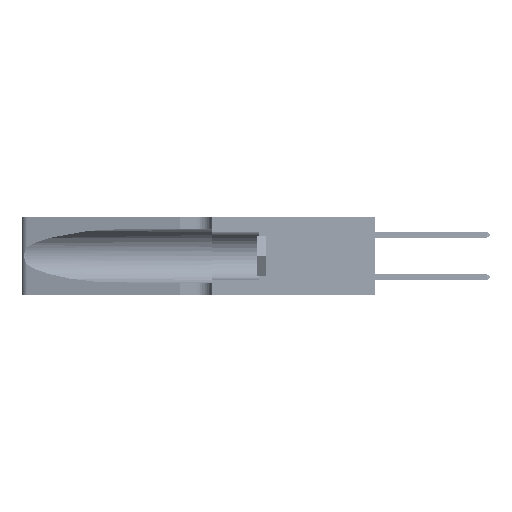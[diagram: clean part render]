
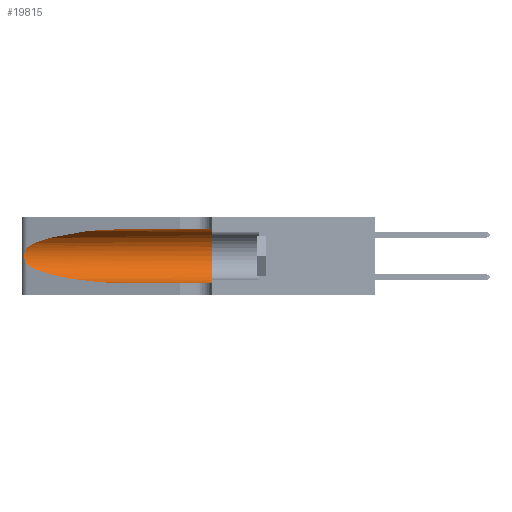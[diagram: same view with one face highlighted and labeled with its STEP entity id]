
A CAD part, left-side view. The second image highlights one B-rep face of the part: STEP entity #19815.
In plain terms, the highlighted cylindrical face has radius 3.308 mm (diameter 6.617 mm), a partial arc.
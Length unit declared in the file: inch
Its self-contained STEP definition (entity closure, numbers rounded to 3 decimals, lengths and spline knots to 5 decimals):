
#216 = DIRECTION ( 'NONE',  ( 0., -1., 0. ) ) ;
#1273 = DIRECTION ( 'NONE',  ( 0., 1., 0. ) ) ;
#1536 = FACE_OUTER_BOUND ( 'NONE', #24089, .T. ) ;
#1923 = VECTOR ( 'NONE', #216, 39.37008 ) ;
#2223 = DIRECTION ( 'NONE',  ( 0., 0., -1. ) ) ;
#2346 = ORIENTED_EDGE ( 'NONE', *, *, #18407, .T. ) ;
#3426 = CARTESIAN_POINT ( 'NONE',  ( 0.25856, 1.23593, 0.16098 ) ) ;
#3861 = CARTESIAN_POINT ( 'NONE',  ( 0.1305, 0.72297, 0.31525 ) ) ;
#4225 = VECTOR ( 'NONE', #5225, 39.37008 ) ;
#5225 = DIRECTION ( 'NONE',  ( 0., -1., 0. ) ) ;
#5783 = LINE ( 'NONE', #40369, #1923 ) ;
#5882 = CARTESIAN_POINT ( 'NONE',  ( 0.1305, 0.72297, 0.05475 ) ) ;
#7433 = VERTEX_POINT ( 'NONE', #36911 ) ;
#7552 = CARTESIAN_POINT ( 'NONE',  ( 0.25639, 1.23186, 0.15144 ) ) ;
#8198 = EDGE_CURVE ( 'NONE', #29718, #7433, #35538, .T. ) ;
#9983 = CARTESIAN_POINT ( 'NONE',  ( 0.25487, 1.22718, 0.22369 ) ) ;
#10720 =( BOUNDED_CURVE ( )  B_SPLINE_CURVE ( 3, ( #15222, #39487, #15399, #43475 ),
 .UNSPECIFIED., .F., .F. ) 
 B_SPLINE_CURVE_WITH_KNOTS ( ( 4, 4 ),
 ( 1.5708, 2.84003 ),
 .UNSPECIFIED. ) 
 CURVE ( )  GEOMETRIC_REPRESENTATION_ITEM ( )  RATIONAL_B_SPLINE_CURVE ( ( 1., 0.87, 0.87, 1. ) ) 
 REPRESENTATION_ITEM ( '' )  );
#11476 = CARTESIAN_POINT ( 'NONE',  ( 0.25487, 1.22718, 0.22369 ) ) ;
#11656 = CARTESIAN_POINT ( 'NONE',  ( 0.25487, 1.22718, 0.14631 ) ) ;
#13279 = AXIS2_PLACEMENT_3D ( 'NONE', #25658, #1273, #29694 ) ;
#13698 = VERTEX_POINT ( 'NONE', #19667 ) ;
#15124 = LINE ( 'NONE', #17372, #4225 ) ;
#15222 = CARTESIAN_POINT ( 'NONE',  ( 0.1305, 0.72297, 0.31525 ) ) ;
#15399 = CARTESIAN_POINT ( 'NONE',  ( 0.2373, 1.15595, 0.28018 ) ) ;
#15605 = CARTESIAN_POINT ( 'NONE',  ( 0.25639, 1.23184, 0.21858 ) ) ;
#15612 = VERTEX_POINT ( 'NONE', #51389 ) ;
#17372 = CARTESIAN_POINT ( 'NONE',  ( 0.1305, 1.61858, 0.05475 ) ) ;
#18407 = EDGE_CURVE ( 'NONE', #13698, #7433, #15124, .T. ) ;
#19667 = CARTESIAN_POINT ( 'NONE',  ( 0.1305, 0.72297, 0.05475 ) ) ;
#19693 = CARTESIAN_POINT ( 'NONE',  ( 0.25854, 1.2359, 0.20912 ) ) ;
#19815 = ADVANCED_FACE ( 'NONE', ( #1536 ), #32636, .F. ) ;
#20430 = ORIENTED_EDGE ( 'NONE', *, *, #29155, .T. ) ;
#21500 = AXIS2_PLACEMENT_3D ( 'NONE', #26624, #22557, #2223 ) ;
#22557 = DIRECTION ( 'NONE',  ( 0., -1., 0. ) ) ;
#23776 = CARTESIAN_POINT ( 'NONE',  ( 0.26075, 1.23896, 0.19203 ) ) ;
#24089 = EDGE_LOOP ( 'NONE', ( #20430, #48212, #42103, #2346, #38307, #40735 ) ) ;
#25658 = CARTESIAN_POINT ( 'NONE',  ( 0.1305, 0.35, 0.185 ) ) ;
#26624 = CARTESIAN_POINT ( 'NONE',  ( 0.1305, 1.61858, 0.185 ) ) ;
#26874 = CARTESIAN_POINT ( 'NONE',  ( 0.1305, 0.35, 0.31525 ) ) ;
#27804 = CARTESIAN_POINT ( 'NONE',  ( 0.26017, 1.23833, 0.17102 ) ) ;
#28047 = VERTEX_POINT ( 'NONE', #3861 ) ;
#29155 = EDGE_CURVE ( 'NONE', #28047, #33355, #10720, .T. ) ;
#29694 = DIRECTION ( 'NONE',  ( 0., 0., 1. ) ) ;
#29718 = VERTEX_POINT ( 'NONE', #26874 ) ;
#30181 = CARTESIAN_POINT ( 'NONE',  ( 0.18966, 0.96281, 0.05475 ) ) ;
#31839 = CARTESIAN_POINT ( 'NONE',  ( 0.25789, 1.23486, 0.15765 ) ) ;
#32636 = CYLINDRICAL_SURFACE ( 'NONE', #21500, 0.13025 ) ;
#33355 = VERTEX_POINT ( 'NONE', #9983 ) ;
#35024 = B_SPLINE_CURVE_WITH_KNOTS ( 'NONE', 3,
 ( #11476, #35686, #15605, #43685, #19693, #47702, #23776, #51707, #27804, #3426, #31839, #7552, #35840, #11656 ),
 .UNSPECIFIED., .F., .F.,
 ( 4, 2, 2, 2, 2, 2, 4 ),
 ( 0., 0.00027, 0.00053, 0.00107, 0.0016, 0.00187, 0.00214 ),
 .UNSPECIFIED. ) ;
#35538 = CIRCLE ( 'NONE', #13279, 0.13025 ) ;
#35686 = CARTESIAN_POINT ( 'NONE',  ( 0.25555, 1.22994, 0.2215 ) ) ;
#35840 = CARTESIAN_POINT ( 'NONE',  ( 0.25555, 1.22993, 0.14849 ) ) ;
#36911 = CARTESIAN_POINT ( 'NONE',  ( 0.1305, 0.35, 0.05475 ) ) ;
#37035 = EDGE_CURVE ( 'NONE', #28047, #29718, #5783, .T. ) ;
#38307 = ORIENTED_EDGE ( 'NONE', *, *, #8198, .F. ) ;
#39487 = CARTESIAN_POINT ( 'NONE',  ( 0.18966, 0.96281, 0.31525 ) ) ;
#40369 = CARTESIAN_POINT ( 'NONE',  ( 0.1305, 1.61858, 0.31525 ) ) ;
#40461 = EDGE_CURVE ( 'NONE', #33355, #15612, #35024, .T. ) ;
#40735 = ORIENTED_EDGE ( 'NONE', *, *, #37035, .F. ) ;
#42103 = ORIENTED_EDGE ( 'NONE', *, *, #50775, .T. ) ;
#43475 = CARTESIAN_POINT ( 'NONE',  ( 0.25487, 1.22718, 0.22369 ) ) ;
#43685 = CARTESIAN_POINT ( 'NONE',  ( 0.25787, 1.23484, 0.2124 ) ) ;
#46052 = CARTESIAN_POINT ( 'NONE',  ( 0.25487, 1.22718, 0.14631 ) ) ;
#47702 = CARTESIAN_POINT ( 'NONE',  ( 0.26018, 1.23835, 0.19895 ) ) ;
#48212 = ORIENTED_EDGE ( 'NONE', *, *, #40461, .T. ) ;
#49709 =( BOUNDED_CURVE ( )  B_SPLINE_CURVE ( 3, ( #46052, #50048, #30181, #5882 ),
 .UNSPECIFIED., .F., .F. ) 
 B_SPLINE_CURVE_WITH_KNOTS ( ( 4, 4 ),
 ( 3.44316, 4.71239 ),
 .UNSPECIFIED. ) 
 CURVE ( )  GEOMETRIC_REPRESENTATION_ITEM ( )  RATIONAL_B_SPLINE_CURVE ( ( 1., 0.87, 0.87, 1. ) ) 
 REPRESENTATION_ITEM ( '' )  );
#50048 = CARTESIAN_POINT ( 'NONE',  ( 0.2373, 1.15595, 0.08982 ) ) ;
#50775 = EDGE_CURVE ( 'NONE', #15612, #13698, #49709, .T. ) ;
#51389 = CARTESIAN_POINT ( 'NONE',  ( 0.25487, 1.22718, 0.14631 ) ) ;
#51707 = CARTESIAN_POINT ( 'NONE',  ( 0.26075, 1.23896, 0.178 ) ) ;
